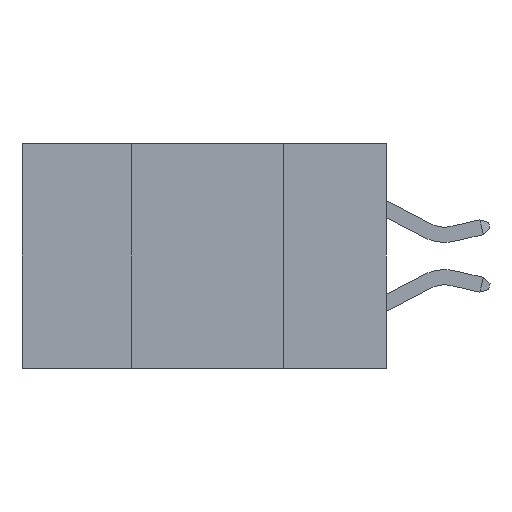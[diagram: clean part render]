
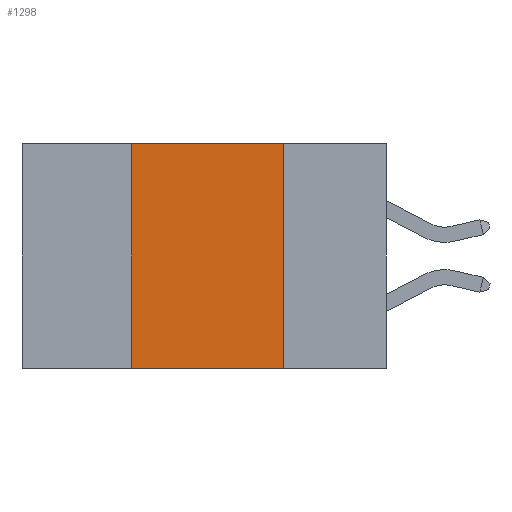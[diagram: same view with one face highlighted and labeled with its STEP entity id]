
A CAD part, left-side view. The second image highlights one B-rep face of the part: STEP entity #1298.
In plain terms, the highlighted planar face has unit normal (-1, 0, 0).
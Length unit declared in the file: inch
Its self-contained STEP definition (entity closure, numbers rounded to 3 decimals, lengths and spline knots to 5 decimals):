
#446 = VERTEX_POINT ( 'NONE', #12789 ) ;
#1298 = ADVANCED_FACE ( 'NONE', ( #10343 ), #9187, .F. ) ;
#1851 = LINE ( 'NONE', #14432, #13826 ) ;
#2130 = CARTESIAN_POINT ( 'NONE',  ( 0., 0.6, -0.37 ) ) ;
#2183 = DIRECTION ( 'NONE',  ( 0., -1., 0. ) ) ;
#2393 = LINE ( 'NONE', #2130, #5265 ) ;
#2853 = LINE ( 'NONE', #6199, #11868 ) ;
#3459 = EDGE_CURVE ( 'NONE', #13049, #446, #2853, .T. ) ;
#3627 = CARTESIAN_POINT ( 'NONE',  ( 0., 0.17, -0.37 ) ) ;
#5030 = ORIENTED_EDGE ( 'NONE', *, *, #12421, .T. ) ;
#5265 = VECTOR ( 'NONE', #2183, 39.37008 ) ;
#6057 = VERTEX_POINT ( 'NONE', #9429 ) ;
#6199 = CARTESIAN_POINT ( 'NONE',  ( 0., 0.6, 0. ) ) ;
#6508 = DIRECTION ( 'NONE',  ( 0., -1., 0. ) ) ;
#7234 = DIRECTION ( 'NONE',  ( 0., 0., -1. ) ) ;
#7827 = ORIENTED_EDGE ( 'NONE', *, *, #3459, .F. ) ;
#8033 = CARTESIAN_POINT ( 'NONE',  ( 0., 0.42, 0. ) ) ;
#8728 = CARTESIAN_POINT ( 'NONE',  ( 0., 0.17, -0.37 ) ) ;
#9187 = PLANE ( 'NONE',  #12105 ) ;
#9241 = CARTESIAN_POINT ( 'NONE',  ( 0., 0.6, 0. ) ) ;
#9429 = CARTESIAN_POINT ( 'NONE',  ( 0., 0.42, -0.37 ) ) ;
#9626 = EDGE_LOOP ( 'NONE', ( #11596, #7827, #13767, #5030 ) ) ;
#10343 = FACE_OUTER_BOUND ( 'NONE', #9626, .T. ) ;
#10948 = EDGE_CURVE ( 'NONE', #6057, #13049, #1851, .T. ) ;
#11596 = ORIENTED_EDGE ( 'NONE', *, *, #13822, .F. ) ;
#11616 = VERTEX_POINT ( 'NONE', #8728 ) ;
#11868 = VECTOR ( 'NONE', #6508, 39.37008 ) ;
#12105 = AXIS2_PLACEMENT_3D ( 'NONE', #9241, #14567, #14564 ) ;
#12421 = EDGE_CURVE ( 'NONE', #6057, #11616, #2393, .T. ) ;
#12789 = CARTESIAN_POINT ( 'NONE',  ( 0., 0.17, 0. ) ) ;
#13049 = VERTEX_POINT ( 'NONE', #8033 ) ;
#13767 = ORIENTED_EDGE ( 'NONE', *, *, #10948, .F. ) ;
#13822 = EDGE_CURVE ( 'NONE', #446, #11616, #14977, .T. ) ;
#13826 = VECTOR ( 'NONE', #13889, 39.37008 ) ;
#13889 = DIRECTION ( 'NONE',  ( 0., 0., 1. ) ) ;
#14399 = VECTOR ( 'NONE', #7234, 39.37008 ) ;
#14432 = CARTESIAN_POINT ( 'NONE',  ( 0., 0.42, -0.37 ) ) ;
#14564 = DIRECTION ( 'NONE',  ( 0., 0., -1. ) ) ;
#14567 = DIRECTION ( 'NONE',  ( 1., 0., 0. ) ) ;
#14977 = LINE ( 'NONE', #3627, #14399 ) ;
